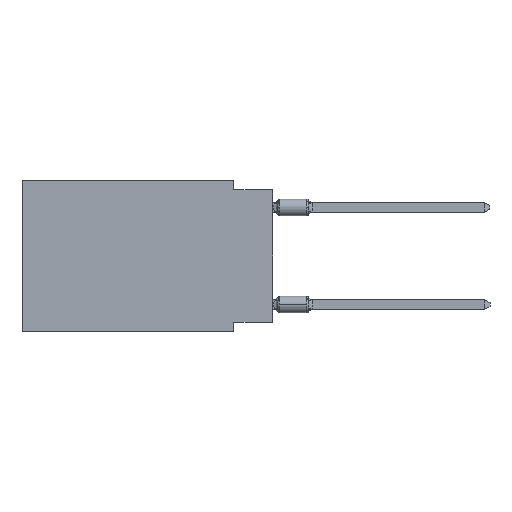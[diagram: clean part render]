
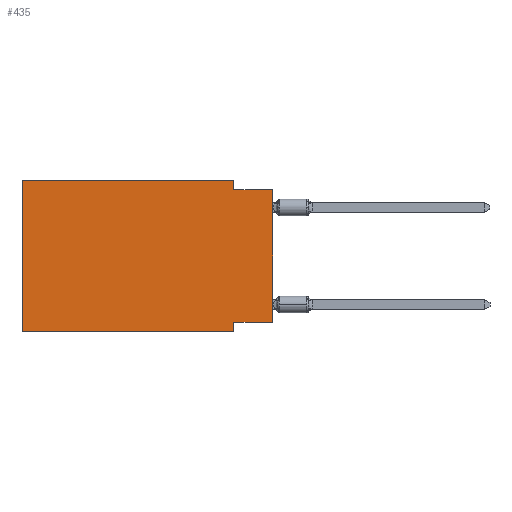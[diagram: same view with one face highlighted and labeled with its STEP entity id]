
A CAD part, left-side view. The second image highlights one B-rep face of the part: STEP entity #435.
In plain terms, the highlighted planar face has unit normal (-1, 0, 0).
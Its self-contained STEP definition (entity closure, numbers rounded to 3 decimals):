
#19 = EDGE_CURVE ( 'NONE', #2935, #5860, #3210, .T. ) ;
#230 = CARTESIAN_POINT ( 'NONE',  ( 0., 0., -0.635 ) ) ;
#435 = ADVANCED_FACE ( 'NONE', ( #1534 ), #486, .F. ) ;
#486 = PLANE ( 'NONE',  #1642 ) ;
#582 = VECTOR ( 'NONE', #8146, 1000. ) ;
#589 = ORIENTED_EDGE ( 'NONE', *, *, #9561, .F. ) ;
#1100 = EDGE_CURVE ( 'NONE', #10845, #12027, #7737, .T. ) ;
#1121 = DIRECTION ( 'NONE',  ( 0., 1., 0. ) ) ;
#1157 = DIRECTION ( 'NONE',  ( 0., -1., 0. ) ) ;
#1534 = FACE_OUTER_BOUND ( 'NONE', #2983, .T. ) ;
#1642 = AXIS2_PLACEMENT_3D ( 'NONE', #14975, #5710, #7000 ) ;
#1973 = VERTEX_POINT ( 'NONE', #13656 ) ;
#2515 = LINE ( 'NONE', #15861, #7516 ) ;
#2693 = DIRECTION ( 'NONE',  ( 0., 0., 1. ) ) ;
#2765 = CARTESIAN_POINT ( 'NONE',  ( 0., 16.383, -9.906 ) ) ;
#2935 = VERTEX_POINT ( 'NONE', #12659 ) ;
#2983 = EDGE_LOOP ( 'NONE', ( #6494, #4476, #16626, #589, #6071, #14122, #16507, #12132 ) ) ;
#3210 = LINE ( 'NONE', #4238, #582 ) ;
#3232 = EDGE_CURVE ( 'NONE', #5860, #14020, #12554, .T. ) ;
#3771 = CARTESIAN_POINT ( 'NONE',  ( 0., 2.54, -9.906 ) ) ;
#3829 = LINE ( 'NONE', #11886, #16528 ) ;
#3945 = CARTESIAN_POINT ( 'NONE',  ( 0., 2.54, -0.635 ) ) ;
#4238 = CARTESIAN_POINT ( 'NONE',  ( 0., 2.54, 0. ) ) ;
#4335 = CARTESIAN_POINT ( 'NONE',  ( 0., 16.383, -9.906 ) ) ;
#4392 = DIRECTION ( 'NONE',  ( 0., -1., 0. ) ) ;
#4476 = ORIENTED_EDGE ( 'NONE', *, *, #3232, .F. ) ;
#4802 = VECTOR ( 'NONE', #4392, 1000. ) ;
#4905 = VERTEX_POINT ( 'NONE', #7158 ) ;
#5710 = DIRECTION ( 'NONE',  ( 1., 0., 0. ) ) ;
#5860 = VERTEX_POINT ( 'NONE', #3945 ) ;
#6071 = ORIENTED_EDGE ( 'NONE', *, *, #11047, .F. ) ;
#6494 = ORIENTED_EDGE ( 'NONE', *, *, #13511, .T. ) ;
#6767 = DIRECTION ( 'NONE',  ( 0., 0., -1. ) ) ;
#7000 = DIRECTION ( 'NONE',  ( 0., 0., -1. ) ) ;
#7158 = CARTESIAN_POINT ( 'NONE',  ( 0., 16.383, 0. ) ) ;
#7277 = VERTEX_POINT ( 'NONE', #4335 ) ;
#7516 = VECTOR ( 'NONE', #1121, 1000. ) ;
#7737 = LINE ( 'NONE', #13272, #11383 ) ;
#8146 = DIRECTION ( 'NONE',  ( 0., 0., -1. ) ) ;
#8920 = CARTESIAN_POINT ( 'NONE',  ( 0., 2.54, -9.271 ) ) ;
#9073 = CARTESIAN_POINT ( 'NONE',  ( 0., 16.383, 0. ) ) ;
#9561 = EDGE_CURVE ( 'NONE', #4905, #2935, #11579, .T. ) ;
#10674 = VECTOR ( 'NONE', #13525, 1000. ) ;
#10845 = VERTEX_POINT ( 'NONE', #8920 ) ;
#11047 = EDGE_CURVE ( 'NONE', #7277, #4905, #15459, .T. ) ;
#11383 = VECTOR ( 'NONE', #6767, 1000. ) ;
#11579 = LINE ( 'NONE', #9073, #14095 ) ;
#11886 = CARTESIAN_POINT ( 'NONE',  ( 0., 0., 0. ) ) ;
#11999 = VECTOR ( 'NONE', #12853, 1000. ) ;
#12027 = VERTEX_POINT ( 'NONE', #3771 ) ;
#12132 = ORIENTED_EDGE ( 'NONE', *, *, #17105, .F. ) ;
#12554 = LINE ( 'NONE', #13666, #4802 ) ;
#12653 = EDGE_CURVE ( 'NONE', #7277, #12027, #13441, .T. ) ;
#12659 = CARTESIAN_POINT ( 'NONE',  ( 0., 2.54, 0. ) ) ;
#12853 = DIRECTION ( 'NONE',  ( 0., 0., 1. ) ) ;
#13272 = CARTESIAN_POINT ( 'NONE',  ( 0., 2.54, -9.906 ) ) ;
#13441 = LINE ( 'NONE', #2765, #10674 ) ;
#13511 = EDGE_CURVE ( 'NONE', #1973, #14020, #3829, .T. ) ;
#13525 = DIRECTION ( 'NONE',  ( 0., -1., 0. ) ) ;
#13656 = CARTESIAN_POINT ( 'NONE',  ( 0., 0., -9.271 ) ) ;
#13666 = CARTESIAN_POINT ( 'NONE',  ( 0., 0., -0.635 ) ) ;
#13815 = CARTESIAN_POINT ( 'NONE',  ( 0., 16.383, 0. ) ) ;
#14020 = VERTEX_POINT ( 'NONE', #230 ) ;
#14095 = VECTOR ( 'NONE', #1157, 1000. ) ;
#14122 = ORIENTED_EDGE ( 'NONE', *, *, #12653, .T. ) ;
#14975 = CARTESIAN_POINT ( 'NONE',  ( 0., 16.383, 0. ) ) ;
#15459 = LINE ( 'NONE', #13815, #11999 ) ;
#15861 = CARTESIAN_POINT ( 'NONE',  ( 0., 0., -9.271 ) ) ;
#16507 = ORIENTED_EDGE ( 'NONE', *, *, #1100, .F. ) ;
#16528 = VECTOR ( 'NONE', #2693, 1000. ) ;
#16626 = ORIENTED_EDGE ( 'NONE', *, *, #19, .F. ) ;
#17105 = EDGE_CURVE ( 'NONE', #1973, #10845, #2515, .T. ) ;
